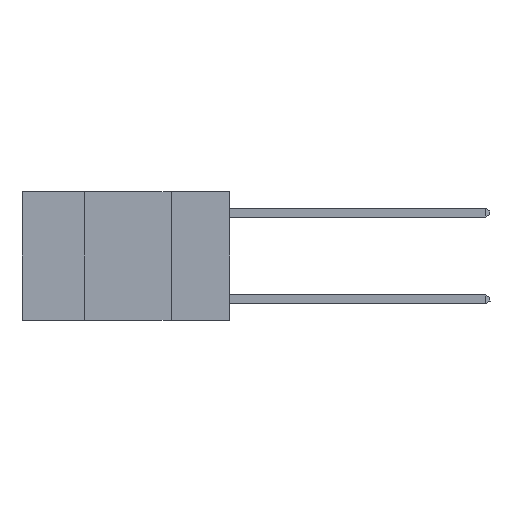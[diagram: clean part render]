
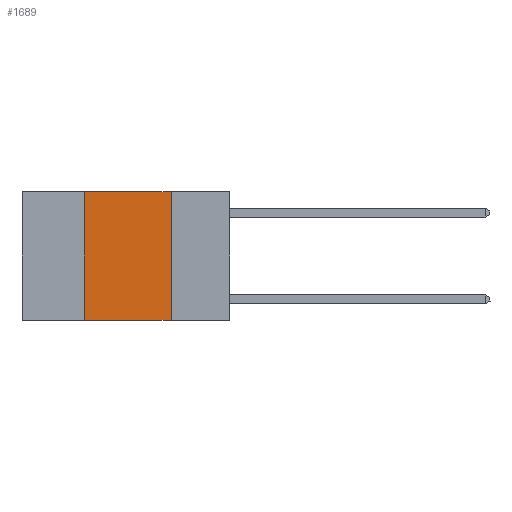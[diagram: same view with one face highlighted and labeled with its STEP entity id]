
A CAD part, left-side view. The second image highlights one B-rep face of the part: STEP entity #1689.
In plain terms, the highlighted planar face has unit normal (-1, 0, 0).
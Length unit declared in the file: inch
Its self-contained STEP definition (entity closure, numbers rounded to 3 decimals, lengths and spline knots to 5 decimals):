
#136 = ORIENTED_EDGE ( 'NONE', *, *, #10586, .F. ) ;
#305 = LINE ( 'NONE', #12283, #3321 ) ;
#1003 = CARTESIAN_POINT ( 'NONE',  ( 0., 0.17, 0. ) ) ;
#1554 = DIRECTION ( 'NONE',  ( 0., -1., 0. ) ) ;
#1689 = ADVANCED_FACE ( 'NONE', ( #9912 ), #2496, .F. ) ;
#1783 = EDGE_CURVE ( 'NONE', #12103, #6480, #5052, .T. ) ;
#1919 = DIRECTION ( 'NONE',  ( 0., -1., 0. ) ) ;
#1965 = VECTOR ( 'NONE', #1919, 39.37008 ) ;
#2033 = VECTOR ( 'NONE', #5294, 39.37008 ) ;
#2496 = PLANE ( 'NONE',  #12719 ) ;
#3321 = VECTOR ( 'NONE', #5431, 39.37008 ) ;
#3882 = ORIENTED_EDGE ( 'NONE', *, *, #1783, .F. ) ;
#4065 = EDGE_CURVE ( 'NONE', #11624, #8408, #305, .T. ) ;
#4140 = LINE ( 'NONE', #7255, #10230 ) ;
#4754 = CARTESIAN_POINT ( 'NONE',  ( 0., 0.17, -0.37 ) ) ;
#4793 = DIRECTION ( 'NONE',  ( 0., 0., -1. ) ) ;
#4986 = LINE ( 'NONE', #11076, #1965 ) ;
#5052 = LINE ( 'NONE', #7223, #2033 ) ;
#5294 = DIRECTION ( 'NONE',  ( 0., 0., 1. ) ) ;
#5330 = ORIENTED_EDGE ( 'NONE', *, *, #7586, .T. ) ;
#5431 = DIRECTION ( 'NONE',  ( 0., 0., -1. ) ) ;
#6255 = CARTESIAN_POINT ( 'NONE',  ( 0., 0.42, 0. ) ) ;
#6480 = VERTEX_POINT ( 'NONE', #6255 ) ;
#7223 = CARTESIAN_POINT ( 'NONE',  ( 0., 0.42, 0. ) ) ;
#7255 = CARTESIAN_POINT ( 'NONE',  ( 0., 0.6, -0.37 ) ) ;
#7586 = EDGE_CURVE ( 'NONE', #12103, #8408, #4140, .T. ) ;
#8408 = VERTEX_POINT ( 'NONE', #4754 ) ;
#9912 = FACE_OUTER_BOUND ( 'NONE', #12402, .T. ) ;
#10230 = VECTOR ( 'NONE', #1554, 39.37008 ) ;
#10510 = CARTESIAN_POINT ( 'NONE',  ( 0., 0.6, 0. ) ) ;
#10586 = EDGE_CURVE ( 'NONE', #6480, #11624, #4986, .T. ) ;
#10991 = CARTESIAN_POINT ( 'NONE',  ( 0., 0.42, -0.37 ) ) ;
#11076 = CARTESIAN_POINT ( 'NONE',  ( 0., 0.6, 0. ) ) ;
#11624 = VERTEX_POINT ( 'NONE', #1003 ) ;
#11663 = DIRECTION ( 'NONE',  ( 1., 0., 0. ) ) ;
#12103 = VERTEX_POINT ( 'NONE', #10991 ) ;
#12283 = CARTESIAN_POINT ( 'NONE',  ( 0., 0.17, 0. ) ) ;
#12402 = EDGE_LOOP ( 'NONE', ( #14255, #136, #3882, #5330 ) ) ;
#12719 = AXIS2_PLACEMENT_3D ( 'NONE', #10510, #11663, #4793 ) ;
#14255 = ORIENTED_EDGE ( 'NONE', *, *, #4065, .F. ) ;
